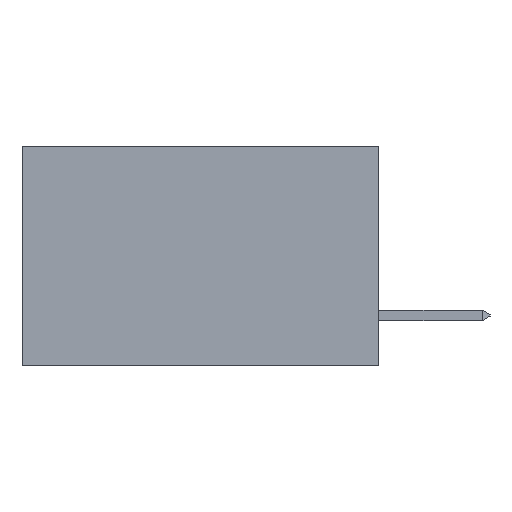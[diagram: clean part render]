
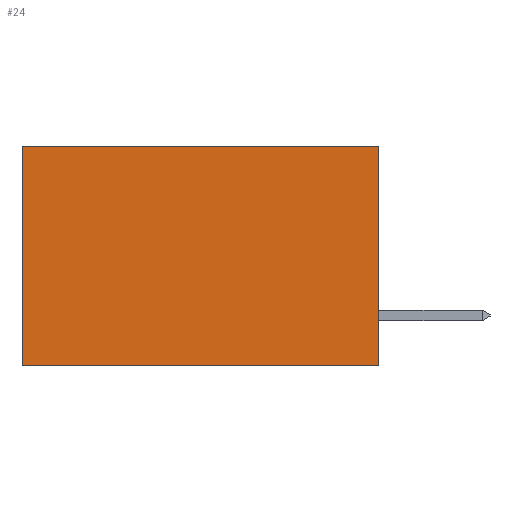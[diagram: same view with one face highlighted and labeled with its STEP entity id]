
A CAD part, left-side view. The second image highlights one B-rep face of the part: STEP entity #24.
In plain terms, the highlighted planar face has unit normal (-1, 0, 0).
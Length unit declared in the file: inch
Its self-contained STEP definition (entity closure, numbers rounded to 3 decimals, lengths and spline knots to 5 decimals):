
#24 = ADVANCED_FACE ( 'NONE', ( #9467 ), #7322, .F. ) ;
#95 = ORIENTED_EDGE ( 'NONE', *, *, #7332, .T. ) ;
#553 = DIRECTION ( 'NONE',  ( 0., 1., 0. ) ) ;
#757 = DIRECTION ( 'NONE',  ( 0., 0., -1. ) ) ;
#872 = VERTEX_POINT ( 'NONE', #3726 ) ;
#1383 = DIRECTION ( 'NONE',  ( 0., 0., -1. ) ) ;
#1385 = CARTESIAN_POINT ( 'NONE',  ( 0.298, 0., 0. ) ) ;
#1667 = DIRECTION ( 'NONE',  ( 1., 0., 0. ) ) ;
#1795 = EDGE_CURVE ( 'NONE', #7887, #9955, #10555, .T. ) ;
#1933 = EDGE_LOOP ( 'NONE', ( #95, #7262, #7534, #4318 ) ) ;
#3179 = EDGE_CURVE ( 'NONE', #7887, #872, #4559, .T. ) ;
#3409 = CARTESIAN_POINT ( 'NONE',  ( 0.298, 0., 0. ) ) ;
#3656 = DIRECTION ( 'NONE',  ( 0., 0., -1. ) ) ;
#3726 = CARTESIAN_POINT ( 'NONE',  ( 0.298, 0.6, 0. ) ) ;
#3979 = VECTOR ( 'NONE', #8030, 39.37008 ) ;
#4318 = ORIENTED_EDGE ( 'NONE', *, *, #3179, .T. ) ;
#4442 = VECTOR ( 'NONE', #3656, 39.37008 ) ;
#4559 = LINE ( 'NONE', #4872, #3979 ) ;
#4567 = CARTESIAN_POINT ( 'NONE',  ( 0.298, 0., 0. ) ) ;
#4872 = CARTESIAN_POINT ( 'NONE',  ( 0.298, 0., 0. ) ) ;
#5138 = CARTESIAN_POINT ( 'NONE',  ( 0.298, 0.6, -0.37 ) ) ;
#5257 = CARTESIAN_POINT ( 'NONE',  ( 0.298, 0., -0.37 ) ) ;
#7027 = LINE ( 'NONE', #10691, #8704 ) ;
#7262 = ORIENTED_EDGE ( 'NONE', *, *, #8528, .F. ) ;
#7322 = PLANE ( 'NONE',  #8365 ) ;
#7332 = EDGE_CURVE ( 'NONE', #872, #10709, #7027, .T. ) ;
#7534 = ORIENTED_EDGE ( 'NONE', *, *, #1795, .F. ) ;
#7887 = VERTEX_POINT ( 'NONE', #4567 ) ;
#8030 = DIRECTION ( 'NONE',  ( 0., 1., 0. ) ) ;
#8193 = LINE ( 'NONE', #5257, #10068 ) ;
#8365 = AXIS2_PLACEMENT_3D ( 'NONE', #1385, #1667, #1383 ) ;
#8528 = EDGE_CURVE ( 'NONE', #9955, #10709, #8193, .T. ) ;
#8704 = VECTOR ( 'NONE', #757, 39.37008 ) ;
#9467 = FACE_OUTER_BOUND ( 'NONE', #1933, .T. ) ;
#9955 = VERTEX_POINT ( 'NONE', #10252 ) ;
#10068 = VECTOR ( 'NONE', #553, 39.37008 ) ;
#10252 = CARTESIAN_POINT ( 'NONE',  ( 0.298, 0., -0.37 ) ) ;
#10555 = LINE ( 'NONE', #3409, #4442 ) ;
#10691 = CARTESIAN_POINT ( 'NONE',  ( 0.298, 0.6, 0. ) ) ;
#10709 = VERTEX_POINT ( 'NONE', #5138 ) ;
